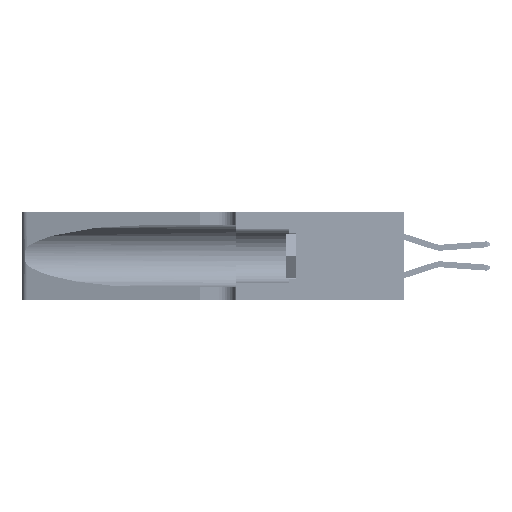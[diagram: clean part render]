
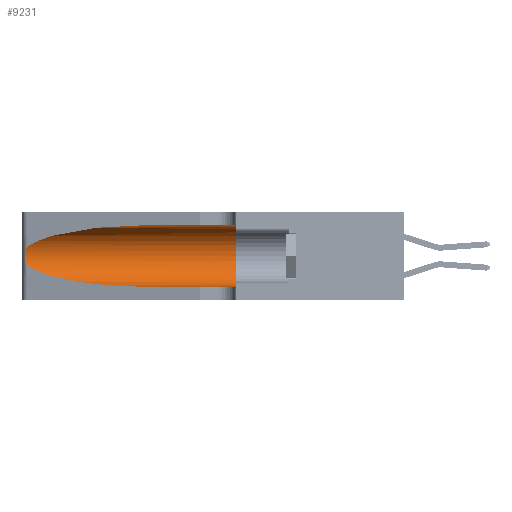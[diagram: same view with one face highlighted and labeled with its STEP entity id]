
A CAD part, left-side view. The second image highlights one B-rep face of the part: STEP entity #9231.
In plain terms, the highlighted cylindrical face has radius 3.308 mm (diameter 6.617 mm), a partial arc.
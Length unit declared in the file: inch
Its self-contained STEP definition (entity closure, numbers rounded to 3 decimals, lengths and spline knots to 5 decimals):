
#825 = DIRECTION ( 'NONE',  ( 0., 0., 1. ) ) ;
#1287 = B_SPLINE_CURVE_WITH_KNOTS ( 'NONE', 3,
 ( #32656, #24290, #16068, #45132, #20273, #49331, #24459, #53501, #28658, #3491, #32822, #7746, #37004, #12050 ),
 .UNSPECIFIED., .F., .F.,
 ( 4, 2, 2, 2, 2, 2, 4 ),
 ( 0., 0.00027, 0.00053, 0.00107, 0.0016, 0.00187, 0.00214 ),
 .UNSPECIFIED. ) ;
#1318 = CARTESIAN_POINT ( 'NONE',  ( 0.25487, 1.22718, 0.22369 ) ) ;
#2735 = ORIENTED_EDGE ( 'NONE', *, *, #51220, .T. ) ;
#3308 = AXIS2_PLACEMENT_3D ( 'NONE', #19865, #48923, #52913 ) ;
#3491 = CARTESIAN_POINT ( 'NONE',  ( 0.25856, 1.23593, 0.16098 ) ) ;
#4432 = EDGE_CURVE ( 'NONE', #39898, #13125, #5436, .T. ) ;
#4507 = AXIS2_PLACEMENT_3D ( 'NONE', #50964, #26107, #825 ) ;
#4615 = CARTESIAN_POINT ( 'NONE',  ( 0.1305, 0.72297, 0.05475 ) ) ;
#4829 = FACE_OUTER_BOUND ( 'NONE', #14630, .T. ) ;
#5095 = CIRCLE ( 'NONE', #4507, 0.13025 ) ;
#5436 =( BOUNDED_CURVE ( )  B_SPLINE_CURVE ( 3, ( #48777, #6988, #11303, #23915 ),
 .UNSPECIFIED., .F., .F. ) 
 B_SPLINE_CURVE_WITH_KNOTS ( ( 4, 4 ),
 ( 1.5708, 2.84003 ),
 .UNSPECIFIED. ) 
 CURVE ( )  GEOMETRIC_REPRESENTATION_ITEM ( )  RATIONAL_B_SPLINE_CURVE ( ( 1., 0.87, 0.87, 1. ) ) 
 REPRESENTATION_ITEM ( '' )  );
#6885 = CARTESIAN_POINT ( 'NONE',  ( 0.2373, 1.15595, 0.08982 ) ) ;
#6988 = CARTESIAN_POINT ( 'NONE',  ( 0.18966, 0.96281, 0.31525 ) ) ;
#7746 = CARTESIAN_POINT ( 'NONE',  ( 0.25639, 1.23186, 0.15144 ) ) ;
#9231 = ADVANCED_FACE ( 'NONE', ( #4829 ), #35622, .F. ) ;
#10790 = LINE ( 'NONE', #53248, #20624 ) ;
#11181 = CARTESIAN_POINT ( 'NONE',  ( 0.18966, 0.96281, 0.05475 ) ) ;
#11303 = CARTESIAN_POINT ( 'NONE',  ( 0.2373, 1.15595, 0.28018 ) ) ;
#12050 = CARTESIAN_POINT ( 'NONE',  ( 0.25487, 1.22718, 0.14631 ) ) ;
#12057 = VERTEX_POINT ( 'NONE', #50356 ) ;
#12697 = ORIENTED_EDGE ( 'NONE', *, *, #22898, .T. ) ;
#13125 = VERTEX_POINT ( 'NONE', #1318 ) ;
#14630 = EDGE_LOOP ( 'NONE', ( #15895, #12697, #2735, #23252, #26012, #49068 ) ) ;
#15895 = ORIENTED_EDGE ( 'NONE', *, *, #4432, .T. ) ;
#15991 = DIRECTION ( 'NONE',  ( 0., -1., 0. ) ) ;
#16068 = CARTESIAN_POINT ( 'NONE',  ( 0.25639, 1.23184, 0.21858 ) ) ;
#16762 = EDGE_CURVE ( 'NONE', #26608, #52925, #10790, .T. ) ;
#17711 = VERTEX_POINT ( 'NONE', #22124 ) ;
#19865 = CARTESIAN_POINT ( 'NONE',  ( 0.1305, 1.61858, 0.185 ) ) ;
#20273 = CARTESIAN_POINT ( 'NONE',  ( 0.25854, 1.2359, 0.20912 ) ) ;
#20624 = VECTOR ( 'NONE', #15991, 39.37008 ) ;
#22124 = CARTESIAN_POINT ( 'NONE',  ( 0.25487, 1.22718, 0.14631 ) ) ;
#22898 = EDGE_CURVE ( 'NONE', #13125, #17711, #1287, .T. ) ;
#23252 = ORIENTED_EDGE ( 'NONE', *, *, #16762, .T. ) ;
#23915 = CARTESIAN_POINT ( 'NONE',  ( 0.25487, 1.22718, 0.22369 ) ) ;
#24290 = CARTESIAN_POINT ( 'NONE',  ( 0.25555, 1.22994, 0.2215 ) ) ;
#24459 = CARTESIAN_POINT ( 'NONE',  ( 0.26075, 1.23896, 0.19203 ) ) ;
#26012 = ORIENTED_EDGE ( 'NONE', *, *, #26670, .F. ) ;
#26107 = DIRECTION ( 'NONE',  ( 0., 1., 0. ) ) ;
#26608 = VERTEX_POINT ( 'NONE', #4615 ) ;
#26670 = EDGE_CURVE ( 'NONE', #12057, #52925, #5095, .T. ) ;
#27631 = CARTESIAN_POINT ( 'NONE',  ( 0.25487, 1.22718, 0.14631 ) ) ;
#28658 = CARTESIAN_POINT ( 'NONE',  ( 0.26017, 1.23833, 0.17102 ) ) ;
#28679 = CARTESIAN_POINT ( 'NONE',  ( 0.1305, 0.72297, 0.31525 ) ) ;
#32656 = CARTESIAN_POINT ( 'NONE',  ( 0.25487, 1.22718, 0.22369 ) ) ;
#32822 = CARTESIAN_POINT ( 'NONE',  ( 0.25789, 1.23486, 0.15765 ) ) ;
#35622 = CYLINDRICAL_SURFACE ( 'NONE', #3308, 0.13025 ) ;
#36050 = EDGE_CURVE ( 'NONE', #39898, #12057, #51339, .T. ) ;
#37004 = CARTESIAN_POINT ( 'NONE',  ( 0.25555, 1.22993, 0.14849 ) ) ;
#39898 = VERTEX_POINT ( 'NONE', #28679 ) ;
#40331 = CARTESIAN_POINT ( 'NONE',  ( 0.1305, 0.72297, 0.05475 ) ) ;
#45132 = CARTESIAN_POINT ( 'NONE',  ( 0.25787, 1.23484, 0.2124 ) ) ;
#45460 = CARTESIAN_POINT ( 'NONE',  ( 0.1305, 1.61858, 0.31525 ) ) ;
#46293 = CARTESIAN_POINT ( 'NONE',  ( 0.1305, 0.35, 0.05475 ) ) ;
#48777 = CARTESIAN_POINT ( 'NONE',  ( 0.1305, 0.72297, 0.31525 ) ) ;
#48923 = DIRECTION ( 'NONE',  ( 0., -1., 0. ) ) ;
#49068 = ORIENTED_EDGE ( 'NONE', *, *, #36050, .F. ) ;
#49331 = CARTESIAN_POINT ( 'NONE',  ( 0.26018, 1.23835, 0.19895 ) ) ;
#49833 = DIRECTION ( 'NONE',  ( 0., -1., 0. ) ) ;
#50027 = VECTOR ( 'NONE', #49833, 39.37008 ) ;
#50356 = CARTESIAN_POINT ( 'NONE',  ( 0.1305, 0.35, 0.31525 ) ) ;
#50964 = CARTESIAN_POINT ( 'NONE',  ( 0.1305, 0.35, 0.185 ) ) ;
#51220 = EDGE_CURVE ( 'NONE', #17711, #26608, #51579, .T. ) ;
#51339 = LINE ( 'NONE', #45460, #50027 ) ;
#51579 =( BOUNDED_CURVE ( )  B_SPLINE_CURVE ( 3, ( #27631, #6885, #11181, #40331 ),
 .UNSPECIFIED., .F., .T. ) 
 B_SPLINE_CURVE_WITH_KNOTS ( ( 4, 4 ),
 ( 3.44316, 4.71239 ),
 .UNSPECIFIED. ) 
 CURVE ( )  GEOMETRIC_REPRESENTATION_ITEM ( )  RATIONAL_B_SPLINE_CURVE ( ( 1., 0.87, 0.87, 1. ) ) 
 REPRESENTATION_ITEM ( '' )  );
#52913 = DIRECTION ( 'NONE',  ( 0., 0., -1. ) ) ;
#52925 = VERTEX_POINT ( 'NONE', #46293 ) ;
#53248 = CARTESIAN_POINT ( 'NONE',  ( 0.1305, 1.61858, 0.05475 ) ) ;
#53501 = CARTESIAN_POINT ( 'NONE',  ( 0.26075, 1.23896, 0.178 ) ) ;
